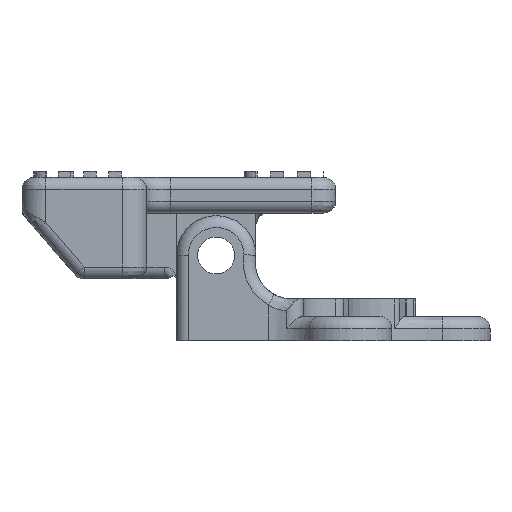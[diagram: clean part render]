
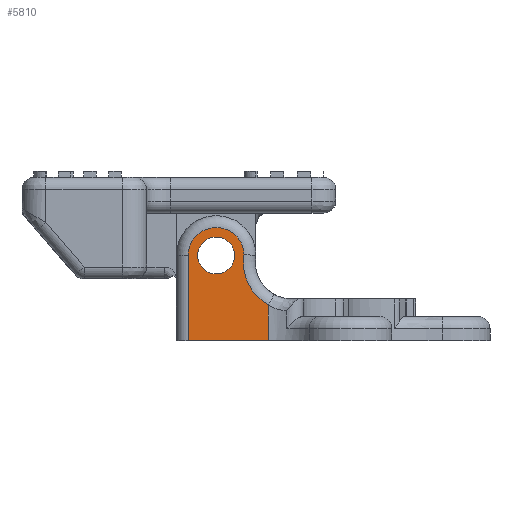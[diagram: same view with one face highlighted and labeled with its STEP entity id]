
A CAD part, left-side view. The second image highlights one B-rep face of the part: STEP entity #5810.
In plain terms, the highlighted planar face has unit normal (-1, 0, 0).
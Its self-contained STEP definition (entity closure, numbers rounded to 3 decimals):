
#103=FACE_BOUND('',#794,.T.);
#126=PLANE('',#6261);
#418=FACE_OUTER_BOUND('',#793,.T.);
#793=EDGE_LOOP('',(#4167,#4168,#4169,#4170,#4171));
#794=EDGE_LOOP('',(#4172));
#1133=LINE('',#8751,#1638);
#1154=LINE('',#9088,#1659);
#1170=LINE('',#9265,#1675);
#1638=VECTOR('',#6877,10.);
#1659=VECTOR('',#7016,10.);
#1675=VECTOR('',#7090,10.);
#2175=CIRCLE('',#6207,2.35);
#2176=CIRCLE('',#6209,4.058);
#2199=CIRCLE('',#6262,1.55);
#2463=VERTEX_POINT('',#8748);
#2464=VERTEX_POINT('',#8750);
#2512=VERTEX_POINT('',#9065);
#2513=VERTEX_POINT('',#9067);
#2514=VERTEX_POINT('',#9082);
#2542=VERTEX_POINT('',#9303);
#3000=EDGE_CURVE('',#2463,#2464,#1133,.F.);
#3068=EDGE_CURVE('',#2512,#2513,#2175,.T.);
#3070=EDGE_CURVE('',#2513,#2514,#2176,.T.);
#3073=EDGE_CURVE('',#2464,#2512,#1154,.T.);
#3114=EDGE_CURVE('',#2514,#2463,#1170,.T.);
#3133=EDGE_CURVE('',#2542,#2542,#2199,.T.);
#4167=ORIENTED_EDGE('',*,*,#3073,.F.);
#4168=ORIENTED_EDGE('',*,*,#3000,.F.);
#4169=ORIENTED_EDGE('',*,*,#3114,.F.);
#4170=ORIENTED_EDGE('',*,*,#3070,.F.);
#4171=ORIENTED_EDGE('',*,*,#3068,.F.);
#4172=ORIENTED_EDGE('',*,*,#3133,.F.);
#5810=ADVANCED_FACE('',(#418,#103),#126,.F.);
#6207=AXIS2_PLACEMENT_3D('',#9068,#7004,#7005);
#6209=AXIS2_PLACEMENT_3D('',#9083,#7008,#7009);
#6261=AXIS2_PLACEMENT_3D('',#9302,#7141,#7142);
#6262=AXIS2_PLACEMENT_3D('',#9304,#7143,#7144);
#6877=DIRECTION('',(0.,-1.,0.));
#7004=DIRECTION('center_axis',(1.,0.,0.));
#7005=DIRECTION('ref_axis',(0.,0.,
1.));
#7008=DIRECTION('center_axis',(-1.,0.,0.));
#7009=DIRECTION('ref_axis',(0.,0.773,-0.635));
#7016=DIRECTION('',(0.,0.,1.));
#7090=DIRECTION('',(0.,0.,-1.));
#7141=DIRECTION('center_axis',(1.,0.,0.));
#7142=DIRECTION('ref_axis',(0.,-1.,0.));
#7143=DIRECTION('center_axis',(-1.,0.,0.));
#7144=DIRECTION('ref_axis',(0.,0.,
1.));
#8748=CARTESIAN_POINT('',(491.066,758.844,-25.283));
#8750=CARTESIAN_POINT('',(491.066,765.583,-25.283));
#8751=CARTESIAN_POINT('',(491.066,748.727,-25.283));
#9065=CARTESIAN_POINT('',(491.066,765.583,-18.13));
#9067=CARTESIAN_POINT('',(491.066,760.885,-18.048));
#9068=CARTESIAN_POINT('Origin',(491.066,763.233,-18.13));
#9082=CARTESIAN_POINT('',(491.066,758.844,-22.275));
#9083=CARTESIAN_POINT('Origin',(491.066,756.883,-18.722));
#9088=CARTESIAN_POINT('',(491.066,765.583,-23.283));
#9265=CARTESIAN_POINT('',(491.066,758.844,-23.283));
#9302=CARTESIAN_POINT('Origin',(491.066,763.906,-23.283));
#9303=CARTESIAN_POINT('',(491.066,763.233,-19.68));
#9304=CARTESIAN_POINT('Origin',(491.066,763.233,-18.13));
